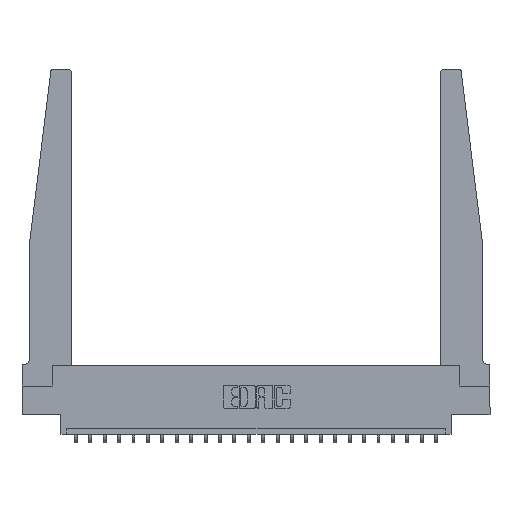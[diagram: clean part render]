
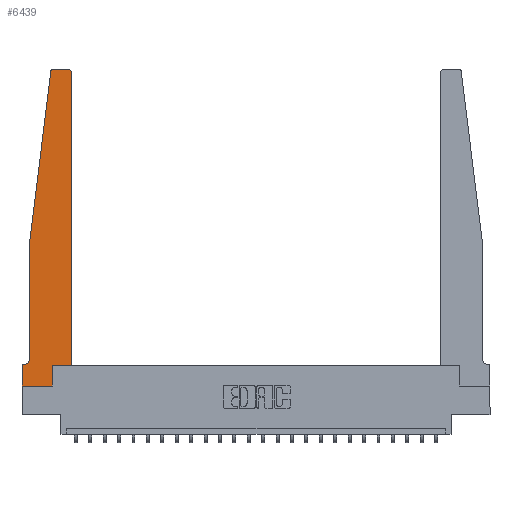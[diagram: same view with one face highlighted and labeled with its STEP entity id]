
A CAD part, top view. The second image highlights one B-rep face of the part: STEP entity #6439.
In plain terms, the highlighted planar face has unit normal (0, 0, 1).
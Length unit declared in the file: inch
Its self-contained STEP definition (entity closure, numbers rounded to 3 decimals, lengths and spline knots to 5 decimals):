
#389 = AXIS2_PLACEMENT_3D ( 'NONE', #11579, #676, #13310 ) ;
#676 = DIRECTION ( 'NONE',  ( 0., 0., 1. ) ) ;
#784 = DIRECTION ( 'NONE',  ( 0., 0., -1. ) ) ;
#1313 = DIRECTION ( 'NONE',  ( 1., 0., 0. ) ) ;
#1472 = CARTESIAN_POINT ( 'NONE',  ( 0., 0., 0.37 ) ) ;
#1474 = EDGE_CURVE ( 'NONE', #17629, #11061, #22018, .T. ) ;
#1478 = CARTESIAN_POINT ( 'NONE',  ( 0.015, 0.1875, 0.37 ) ) ;
#1647 = CARTESIAN_POINT ( 'NONE',  ( 0., 0., 0.37 ) ) ;
#1932 = DIRECTION ( 'NONE',  ( 0., 1., 0. ) ) ;
#2705 = ORIENTED_EDGE ( 'NONE', *, *, #7167, .T. ) ;
#3106 = VERTEX_POINT ( 'NONE', #19750 ) ;
#3309 = EDGE_CURVE ( 'NONE', #16651, #17629, #9775, .T. ) ;
#3610 = VECTOR ( 'NONE', #1313, 39.37008 ) ;
#3841 = VECTOR ( 'NONE', #5196, 39.37008 ) ;
#4038 = CARTESIAN_POINT ( 'NONE',  ( 0.395, 2.72, 0.37 ) ) ;
#4091 = EDGE_CURVE ( 'NONE', #20572, #14021, #12465, .T. ) ;
#4398 = VECTOR ( 'NONE', #12070, 39.37008 ) ;
#4487 = FACE_OUTER_BOUND ( 'NONE', #12495, .T. ) ;
#4523 = VERTEX_POINT ( 'NONE', #16838 ) ;
#4737 = ORIENTED_EDGE ( 'NONE', *, *, #11222, .T. ) ;
#4749 = LINE ( 'NONE', #21844, #23158 ) ;
#4955 = CARTESIAN_POINT ( 'NONE',  ( 0.425, 0.18, 0.37 ) ) ;
#5196 = DIRECTION ( 'NONE',  ( 1., 0., 0. ) ) ;
#5623 = EDGE_CURVE ( 'NONE', #14021, #7372, #6530, .T. ) ;
#5724 = AXIS2_PLACEMENT_3D ( 'NONE', #4038, #16558, #5878 ) ;
#5878 = DIRECTION ( 'NONE',  ( 1., 0., 0. ) ) ;
#6439 = ADVANCED_FACE ( 'NONE', ( #4487 ), #8654, .T. ) ;
#6530 = CIRCLE ( 'NONE', #5724, 0.03 ) ;
#6642 = CARTESIAN_POINT ( 'NONE',  ( 0.065, 1.25, 0.37 ) ) ;
#7167 = EDGE_CURVE ( 'NONE', #11061, #17674, #4749, .T. ) ;
#7372 = VERTEX_POINT ( 'NONE', #16973 ) ;
#7764 = VECTOR ( 'NONE', #22481, 39.37008 ) ;
#8173 = DIRECTION ( 'NONE',  ( -0.122, -0.992, 0. ) ) ;
#8470 = CARTESIAN_POINT ( 'NONE',  ( 0.2605, 0., 0.37 ) ) ;
#8528 = CARTESIAN_POINT ( 'NONE',  ( 0.25, 2.75, 0.37 ) ) ;
#8654 = PLANE ( 'NONE',  #16768 ) ;
#9775 = CIRCLE ( 'NONE', #21985, 0.05 ) ;
#9780 = CIRCLE ( 'NONE', #389, 0.03 ) ;
#9865 = CARTESIAN_POINT ( 'NONE',  ( 0.425, 0.18, 0.37 ) ) ;
#10191 = VECTOR ( 'NONE', #1932, 39.37008 ) ;
#10336 = EDGE_CURVE ( 'NONE', #7372, #3106, #22841, .T. ) ;
#10434 = DIRECTION ( 'NONE',  ( 0., 0., 1. ) ) ;
#11002 = CARTESIAN_POINT ( 'NONE',  ( 0.2605, 0.18, 0.37 ) ) ;
#11061 = VERTEX_POINT ( 'NONE', #19881 ) ;
#11222 = EDGE_CURVE ( 'NONE', #3106, #14853, #9780, .T. ) ;
#11457 = CARTESIAN_POINT ( 'NONE',  ( 0.24675, 2.72367, 0.37 ) ) ;
#11579 = CARTESIAN_POINT ( 'NONE',  ( 0.27653, 2.72, 0.37 ) ) ;
#11677 = CARTESIAN_POINT ( 'NONE',  ( 0.015, 0.2375, 0.37 ) ) ;
#11787 = ORIENTED_EDGE ( 'NONE', *, *, #3309, .T. ) ;
#11852 = CARTESIAN_POINT ( 'NONE',  ( 0.425, 0.18, 0.37 ) ) ;
#12070 = DIRECTION ( 'NONE',  ( -1., 0., 0. ) ) ;
#12465 = LINE ( 'NONE', #11852, #7764 ) ;
#12495 = EDGE_LOOP ( 'NONE', ( #18711, #4737, #19549, #20122, #11787, #21257, #2705, #21804, #12864, #22335, #18181, #14532 ) ) ;
#12864 = ORIENTED_EDGE ( 'NONE', *, *, #21652, .T. ) ;
#12893 = LINE ( 'NONE', #16978, #21285 ) ;
#12942 = DIRECTION ( 'NONE',  ( 0., -1., 0. ) ) ;
#12974 = VERTEX_POINT ( 'NONE', #8470 ) ;
#13164 = VERTEX_POINT ( 'NONE', #17835 ) ;
#13186 = DIRECTION ( 'NONE',  ( -1., 0., 0. ) ) ;
#13310 = DIRECTION ( 'NONE',  ( 1., 0., 0. ) ) ;
#13350 = VECTOR ( 'NONE', #15481, 39.37008 ) ;
#13409 = DIRECTION ( 'NONE',  ( -1., 0., 0. ) ) ;
#14021 = VERTEX_POINT ( 'NONE', #16445 ) ;
#14317 = EDGE_CURVE ( 'NONE', #4523, #16651, #18120, .T. ) ;
#14532 = ORIENTED_EDGE ( 'NONE', *, *, #5623, .T. ) ;
#14831 = LINE ( 'NONE', #11002, #10191 ) ;
#14853 = VERTEX_POINT ( 'NONE', #11457 ) ;
#15044 = CARTESIAN_POINT ( 'NONE',  ( 0.065, 0.2375, 0.37 ) ) ;
#15481 = DIRECTION ( 'NONE',  ( 0., -1., 0. ) ) ;
#16445 = CARTESIAN_POINT ( 'NONE',  ( 0.425, 2.72, 0.37 ) ) ;
#16558 = DIRECTION ( 'NONE',  ( 0., 0., 1. ) ) ;
#16651 = VERTEX_POINT ( 'NONE', #15044 ) ;
#16768 = AXIS2_PLACEMENT_3D ( 'NONE', #21082, #10434, #22826 ) ;
#16838 = CARTESIAN_POINT ( 'NONE',  ( 0.065, 1.25, 0.37 ) ) ;
#16973 = CARTESIAN_POINT ( 'NONE',  ( 0.395, 2.75, 0.37 ) ) ;
#16978 = CARTESIAN_POINT ( 'NONE',  ( 0.065, 1.25, 0.37 ) ) ;
#17629 = VERTEX_POINT ( 'NONE', #1478 ) ;
#17674 = VERTEX_POINT ( 'NONE', #1647 ) ;
#17835 = CARTESIAN_POINT ( 'NONE',  ( 0.2605, 0.18, 0.37 ) ) ;
#17921 = LINE ( 'NONE', #4955, #3610 ) ;
#18109 = EDGE_CURVE ( 'NONE', #14853, #4523, #12893, .T. ) ;
#18120 = LINE ( 'NONE', #6642, #13350 ) ;
#18149 = LINE ( 'NONE', #1472, #3841 ) ;
#18181 = ORIENTED_EDGE ( 'NONE', *, *, #4091, .T. ) ;
#18338 = EDGE_CURVE ( 'NONE', #13164, #20572, #17921, .T. ) ;
#18425 = CARTESIAN_POINT ( 'NONE',  ( 0.065, 0.1875, 0.37 ) ) ;
#18711 = ORIENTED_EDGE ( 'NONE', *, *, #10336, .T. ) ;
#19549 = ORIENTED_EDGE ( 'NONE', *, *, #18109, .T. ) ;
#19750 = CARTESIAN_POINT ( 'NONE',  ( 0.27653, 2.75, 0.37 ) ) ;
#19881 = CARTESIAN_POINT ( 'NONE',  ( 0., 0.1875, 0.37 ) ) ;
#20122 = ORIENTED_EDGE ( 'NONE', *, *, #14317, .T. ) ;
#20190 = EDGE_CURVE ( 'NONE', #17674, #12974, #18149, .T. ) ;
#20572 = VERTEX_POINT ( 'NONE', #9865 ) ;
#21082 = CARTESIAN_POINT ( 'NONE',  ( 0., 0.1875, 0.37 ) ) ;
#21257 = ORIENTED_EDGE ( 'NONE', *, *, #1474, .T. ) ;
#21285 = VECTOR ( 'NONE', #8173, 39.37008 ) ;
#21479 = VECTOR ( 'NONE', #13186, 39.37008 ) ;
#21652 = EDGE_CURVE ( 'NONE', #12974, #13164, #14831, .T. ) ;
#21804 = ORIENTED_EDGE ( 'NONE', *, *, #20190, .T. ) ;
#21844 = CARTESIAN_POINT ( 'NONE',  ( 0., 0., 0.37 ) ) ;
#21985 = AXIS2_PLACEMENT_3D ( 'NONE', #11677, #784, #13409 ) ;
#22018 = LINE ( 'NONE', #18425, #21479 ) ;
#22335 = ORIENTED_EDGE ( 'NONE', *, *, #18338, .T. ) ;
#22481 = DIRECTION ( 'NONE',  ( 0., 1., 0. ) ) ;
#22826 = DIRECTION ( 'NONE',  ( 1., 0., 0. ) ) ;
#22841 = LINE ( 'NONE', #8528, #4398 ) ;
#23158 = VECTOR ( 'NONE', #12942, 39.37008 ) ;
